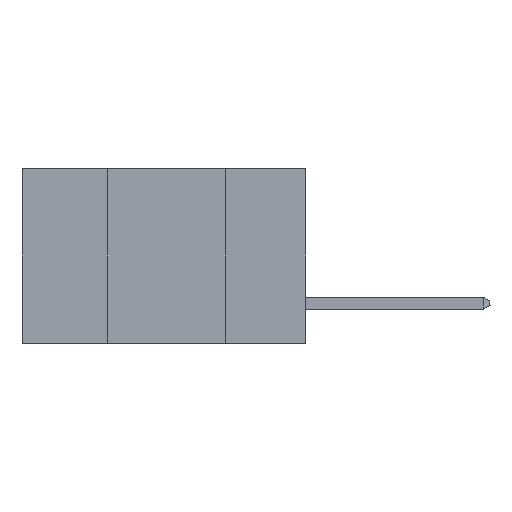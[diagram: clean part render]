
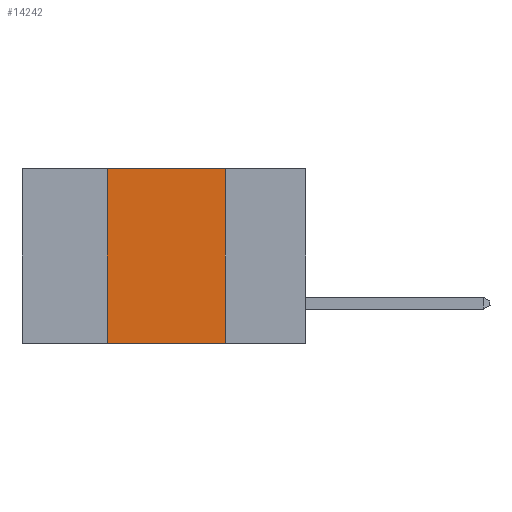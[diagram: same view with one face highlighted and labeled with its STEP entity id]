
A CAD part, left-side view. The second image highlights one B-rep face of the part: STEP entity #14242.
In plain terms, the highlighted planar face has unit normal (-1, 0, 0).
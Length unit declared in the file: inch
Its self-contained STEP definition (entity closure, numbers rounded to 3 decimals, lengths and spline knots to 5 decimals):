
#681 = CARTESIAN_POINT ( 'NONE',  ( 0., 0.6, 0. ) ) ;
#2043 = FACE_OUTER_BOUND ( 'NONE', #14181, .T. ) ;
#3300 = VERTEX_POINT ( 'NONE', #14103 ) ;
#3790 = DIRECTION ( 'NONE',  ( 0., -1., 0. ) ) ;
#3846 = VECTOR ( 'NONE', #18634, 39.37008 ) ;
#4189 = CARTESIAN_POINT ( 'NONE',  ( 0., 0.17, -0.37 ) ) ;
#5129 = ORIENTED_EDGE ( 'NONE', *, *, #8314, .F. ) ;
#5286 = VERTEX_POINT ( 'NONE', #17320 ) ;
#5512 = VECTOR ( 'NONE', #10529, 39.37008 ) ;
#5640 = CARTESIAN_POINT ( 'NONE',  ( 0., 0.17, 0. ) ) ;
#5701 = DIRECTION ( 'NONE',  ( 1., 0., 0. ) ) ;
#5781 = LINE ( 'NONE', #681, #20267 ) ;
#5953 = ORIENTED_EDGE ( 'NONE', *, *, #6256, .F. ) ;
#6256 = EDGE_CURVE ( 'NONE', #3300, #17751, #8238, .T. ) ;
#6576 = VECTOR ( 'NONE', #10159, 39.37008 ) ;
#7049 = PLANE ( 'NONE',  #16544 ) ;
#7314 = CARTESIAN_POINT ( 'NONE',  ( 0., 0.42, -0.37 ) ) ;
#8238 = LINE ( 'NONE', #5640, #3846 ) ;
#8314 = EDGE_CURVE ( 'NONE', #18345, #5286, #14565, .T. ) ;
#9411 = ORIENTED_EDGE ( 'NONE', *, *, #17620, .T. ) ;
#10159 = DIRECTION ( 'NONE',  ( 0., -1., 0. ) ) ;
#10529 = DIRECTION ( 'NONE',  ( 0., 0., 1. ) ) ;
#11903 = CARTESIAN_POINT ( 'NONE',  ( 0., 0.42, 0. ) ) ;
#14103 = CARTESIAN_POINT ( 'NONE',  ( 0., 0.17, 0. ) ) ;
#14181 = EDGE_LOOP ( 'NONE', ( #5953, #18242, #5129, #9411 ) ) ;
#14185 = LINE ( 'NONE', #16649, #6576 ) ;
#14242 = ADVANCED_FACE ( 'NONE', ( #2043 ), #7049, .F. ) ;
#14565 = LINE ( 'NONE', #11903, #5512 ) ;
#16544 = AXIS2_PLACEMENT_3D ( 'NONE', #19776, #5701, #19835 ) ;
#16649 = CARTESIAN_POINT ( 'NONE',  ( 0., 0.6, -0.37 ) ) ;
#17320 = CARTESIAN_POINT ( 'NONE',  ( 0., 0.42, 0. ) ) ;
#17620 = EDGE_CURVE ( 'NONE', #18345, #17751, #14185, .T. ) ;
#17751 = VERTEX_POINT ( 'NONE', #4189 ) ;
#18242 = ORIENTED_EDGE ( 'NONE', *, *, #19589, .F. ) ;
#18345 = VERTEX_POINT ( 'NONE', #7314 ) ;
#18634 = DIRECTION ( 'NONE',  ( 0., 0., -1. ) ) ;
#19589 = EDGE_CURVE ( 'NONE', #5286, #3300, #5781, .T. ) ;
#19776 = CARTESIAN_POINT ( 'NONE',  ( 0., 0.6, 0. ) ) ;
#19835 = DIRECTION ( 'NONE',  ( 0., 0., -1. ) ) ;
#20267 = VECTOR ( 'NONE', #3790, 39.37008 ) ;
